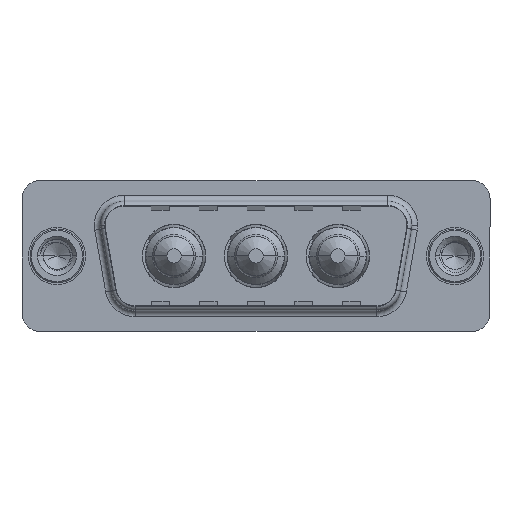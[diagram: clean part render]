
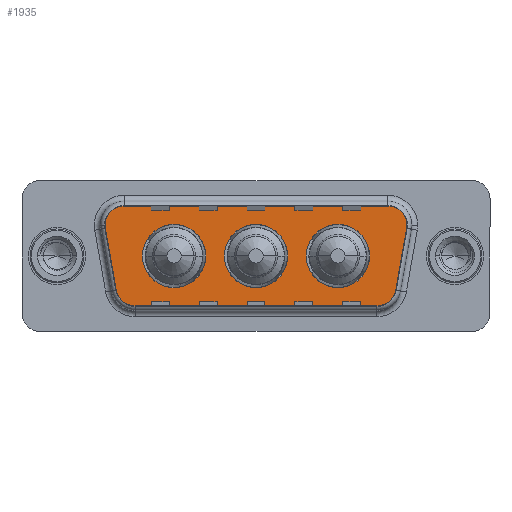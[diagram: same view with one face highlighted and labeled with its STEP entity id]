
A CAD part, top view. The second image highlights one B-rep face of the part: STEP entity #1935.
In plain terms, the highlighted planar face has unit normal (0, 0, 1).
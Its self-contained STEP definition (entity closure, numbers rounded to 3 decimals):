
#6 = VERTEX_POINT ( 'NONE', #1034 ) ;
#29 = ORIENTED_EDGE ( 'NONE', *, *, #5355, .T. ) ;
#164 = ORIENTED_EDGE ( 'NONE', *, *, #4156, .F. ) ;
#382 = EDGE_CURVE ( 'NONE', #2594, #4807, #12062, .T. ) ;
#663 = AXIS2_PLACEMENT_3D ( 'NONE', #7230, #15959, #8486 ) ;
#745 = ORIENTED_EDGE ( 'NONE', *, *, #11146, .T. ) ;
#750 = FACE_BOUND ( 'NONE', #5321, .T. ) ;
#793 = CARTESIAN_POINT ( 'NONE',  ( 29.859, 2.553, 0. ) ) ;
#1022 = CIRCLE ( 'NONE', #11190, 2.65 ) ;
#1034 = CARTESIAN_POINT ( 'NONE',  ( 19.3, 0., 0. ) ) ;
#1224 = EDGE_CURVE ( 'NONE', #3193, #6191, #15080, .T. ) ;
#1246 = DIRECTION ( 'NONE',  ( 0., 0., 1. ) ) ;
#1613 = CARTESIAN_POINT ( 'NONE',  ( 9.8, 0., 0. ) ) ;
#1647 = DIRECTION ( 'NONE',  ( -1., 0., 0. ) ) ;
#1658 = CARTESIAN_POINT ( 'NONE',  ( 16.65, 0., 0. ) ) ;
#1691 = VECTOR ( 'NONE', #12616, 1000. ) ;
#1693 = DIRECTION ( 'NONE',  ( 1., 0., 0. ) ) ;
#1715 = CARTESIAN_POINT ( 'NONE',  ( 6.434, -2.9, 0. ) ) ;
#1935 = ADVANCED_FACE ( 'NONE', ( #750, #4996, #11005, #13918 ), #15653, .T. ) ;
#2195 = CARTESIAN_POINT ( 'NONE',  ( 5.411, 2.9, 0. ) ) ;
#2594 = VERTEX_POINT ( 'NONE', #4792 ) ;
#2639 = VERTEX_POINT ( 'NONE', #12435 ) ;
#2667 = ORIENTED_EDGE ( 'NONE', *, *, #382, .T. ) ;
#2906 = DIRECTION ( 'NONE',  ( 1., 0., 0. ) ) ;
#2926 = CIRCLE ( 'NONE', #663, 2.65 ) ;
#2974 = ORIENTED_EDGE ( 'NONE', *, *, #1224, .T. ) ;
#3021 = EDGE_CURVE ( 'NONE', #6468, #2594, #11612, .T. ) ;
#3032 = DIRECTION ( 'NONE',  ( -1., 0., 0. ) ) ;
#3085 = CARTESIAN_POINT ( 'NONE',  ( 23.5, 0., 0. ) ) ;
#3167 = VERTEX_POINT ( 'NONE', #7704 ) ;
#3189 = CARTESIAN_POINT ( 'NONE',  ( 23.5, 0., 0. ) ) ;
#3193 = VERTEX_POINT ( 'NONE', #12414 ) ;
#3243 = EDGE_LOOP ( 'NONE', ( #8648, #11175 ) ) ;
#3401 = CARTESIAN_POINT ( 'NONE',  ( 6.434, -4.9, 0. ) ) ;
#3408 = CARTESIAN_POINT ( 'NONE',  ( 20.85, 0., 0. ) ) ;
#3487 = DIRECTION ( 'NONE',  ( 1., 0., 0. ) ) ;
#3648 = CARTESIAN_POINT ( 'NONE',  ( 26.866, -2.9, 0. ) ) ;
#3726 = ORIENTED_EDGE ( 'NONE', *, *, #3021, .T. ) ;
#3740 = DIRECTION ( 'NONE',  ( 1., 0., 0. ) ) ;
#3808 = AXIS2_PLACEMENT_3D ( 'NONE', #2195, #11163, #3487 ) ;
#3938 = EDGE_LOOP ( 'NONE', ( #3726, #2667, #745, #2974, #15783, #15108, #29, #9210, #5083 ) ) ;
#4156 = EDGE_CURVE ( 'NONE', #6, #4825, #15232, .T. ) ;
#4379 = DIRECTION ( 'NONE',  ( 1., 0., 0. ) ) ;
#4480 = DIRECTION ( 'NONE',  ( 1., 0., 0. ) ) ;
#4767 = VERTEX_POINT ( 'NONE', #15723 ) ;
#4792 = CARTESIAN_POINT ( 'NONE',  ( 28.836, -3.247, 0. ) ) ;
#4807 = VERTEX_POINT ( 'NONE', #793 ) ;
#4825 = VERTEX_POINT ( 'NONE', #14793 ) ;
#4984 = CARTESIAN_POINT ( 'NONE',  ( 6.434, -4.9, 0. ) ) ;
#4996 = FACE_BOUND ( 'NONE', #14342, .T. ) ;
#5043 = CARTESIAN_POINT ( 'NONE',  ( 27.889, 2.9, 0. ) ) ;
#5083 = ORIENTED_EDGE ( 'NONE', *, *, #11165, .T. ) ;
#5124 = LINE ( 'NONE', #11335, #1691 ) ;
#5321 = EDGE_LOOP ( 'NONE', ( #164, #16284 ) ) ;
#5355 = EDGE_CURVE ( 'NONE', #2639, #13304, #5124, .T. ) ;
#5622 = CIRCLE ( 'NONE', #8593, 2.65 ) ;
#5738 = DIRECTION ( 'NONE',  ( 0.174, 0.985, 0. ) ) ;
#5825 = CARTESIAN_POINT ( 'NONE',  ( 26.866, -4.9, 0. ) ) ;
#5869 = AXIS2_PLACEMENT_3D ( 'NONE', #1658, #13977, #13877 ) ;
#6157 = CARTESIAN_POINT ( 'NONE',  ( 16.65, 0., 0. ) ) ;
#6191 = VERTEX_POINT ( 'NONE', #12926 ) ;
#6260 = ORIENTED_EDGE ( 'NONE', *, *, #7836, .F. ) ;
#6334 = DIRECTION ( 'NONE',  ( -1., 0., 0. ) ) ;
#6335 = VERTEX_POINT ( 'NONE', #12010 ) ;
#6468 = VERTEX_POINT ( 'NONE', #5825 ) ;
#6509 = VERTEX_POINT ( 'NONE', #3408 ) ;
#6524 = CARTESIAN_POINT ( 'NONE',  ( 26.866, -2.9, 0. ) ) ;
#6906 = CIRCLE ( 'NONE', #15013, 2.65 ) ;
#6947 = DIRECTION ( 'NONE',  ( 0., 0., 1. ) ) ;
#7230 = CARTESIAN_POINT ( 'NONE',  ( 9.8, 0., 0. ) ) ;
#7366 = LINE ( 'NONE', #4984, #13691 ) ;
#7403 = EDGE_CURVE ( 'NONE', #6191, #4767, #14151, .T. ) ;
#7454 = DIRECTION ( 'NONE',  ( 1., 0., 0. ) ) ;
#7704 = CARTESIAN_POINT ( 'NONE',  ( 12.45, 0., 0. ) ) ;
#7747 = CARTESIAN_POINT ( 'NONE',  ( 4.464, -3.247, 0. ) ) ;
#7836 = EDGE_CURVE ( 'NONE', #6509, #12329, #5622, .T. ) ;
#7863 = AXIS2_PLACEMENT_3D ( 'NONE', #3648, #1246, #1693 ) ;
#8486 = DIRECTION ( 'NONE',  ( 1., 0., 0. ) ) ;
#8502 = CARTESIAN_POINT ( 'NONE',  ( 29.859, 2.553, 0. ) ) ;
#8593 = AXIS2_PLACEMENT_3D ( 'NONE', #3189, #12156, #4480 ) ;
#8648 = ORIENTED_EDGE ( 'NONE', *, *, #11596, .F. ) ;
#9058 = VECTOR ( 'NONE', #5738, 1000. ) ;
#9206 = AXIS2_PLACEMENT_3D ( 'NONE', #6524, #11009, #16078 ) ;
#9210 = ORIENTED_EDGE ( 'NONE', *, *, #15912, .T. ) ;
#9809 = VERTEX_POINT ( 'NONE', #3401 ) ;
#10577 = DIRECTION ( 'NONE',  ( 0., 0., 1. ) ) ;
#10643 = CARTESIAN_POINT ( 'NONE',  ( 26.15, 0., 0. ) ) ;
#10671 = AXIS2_PLACEMENT_3D ( 'NONE', #1715, #10700, #3032 ) ;
#10700 = DIRECTION ( 'NONE',  ( 0., 0., 1. ) ) ;
#10840 = VECTOR ( 'NONE', #12672, 1000. ) ;
#11005 = FACE_BOUND ( 'NONE', #3243, .T. ) ;
#11009 = DIRECTION ( 'NONE',  ( 0., 0., 1. ) ) ;
#11146 = EDGE_CURVE ( 'NONE', #4807, #3193, #11159, .T. ) ;
#11159 = CIRCLE ( 'NONE', #12802, 2. ) ;
#11163 = DIRECTION ( 'NONE',  ( 0., 0., 1. ) ) ;
#11165 = EDGE_CURVE ( 'NONE', #9809, #6468, #7366, .T. ) ;
#11175 = ORIENTED_EDGE ( 'NONE', *, *, #14110, .F. ) ;
#11190 = AXIS2_PLACEMENT_3D ( 'NONE', #1613, #10577, #2906 ) ;
#11335 = CARTESIAN_POINT ( 'NONE',  ( 3.441, 2.553, 0. ) ) ;
#11402 = CARTESIAN_POINT ( 'NONE',  ( 5.411, 4.9, 0. ) ) ;
#11596 = EDGE_CURVE ( 'NONE', #3167, #6335, #2926, .T. ) ;
#11612 = CIRCLE ( 'NONE', #9206, 2. ) ;
#11948 = EDGE_CURVE ( 'NONE', #4767, #2639, #14634, .T. ) ;
#12010 = CARTESIAN_POINT ( 'NONE',  ( 7.15, 0., 0. ) ) ;
#12062 = LINE ( 'NONE', #8502, #9058 ) ;
#12064 = DIRECTION ( 'NONE',  ( 0., 0., 1. ) ) ;
#12156 = DIRECTION ( 'NONE',  ( 0., 0., 1. ) ) ;
#12329 = VERTEX_POINT ( 'NONE', #10643 ) ;
#12378 = AXIS2_PLACEMENT_3D ( 'NONE', #3085, #12064, #4379 ) ;
#12414 = CARTESIAN_POINT ( 'NONE',  ( 29.889, 2.9, 0. ) ) ;
#12435 = CARTESIAN_POINT ( 'NONE',  ( 3.441, 2.553, 0. ) ) ;
#12616 = DIRECTION ( 'NONE',  ( 0.174, -0.985, 0. ) ) ;
#12672 = DIRECTION ( 'NONE',  ( -1., 0., 0. ) ) ;
#12802 = AXIS2_PLACEMENT_3D ( 'NONE', #5043, #13910, #6334 ) ;
#12926 = CARTESIAN_POINT ( 'NONE',  ( 27.889, 4.9, 0. ) ) ;
#13304 = VERTEX_POINT ( 'NONE', #7747 ) ;
#13425 = CARTESIAN_POINT ( 'NONE',  ( 27.889, 2.9, 0. ) ) ;
#13691 = VECTOR ( 'NONE', #3740, 1000. ) ;
#13877 = DIRECTION ( 'NONE',  ( 1., 0., 0. ) ) ;
#13910 = DIRECTION ( 'NONE',  ( 0., 0., 1. ) ) ;
#13918 = FACE_OUTER_BOUND ( 'NONE', #3938, .T. ) ;
#13960 = CIRCLE ( 'NONE', #12378, 2.65 ) ;
#13977 = DIRECTION ( 'NONE',  ( 0., 0., 1. ) ) ;
#14110 = EDGE_CURVE ( 'NONE', #6335, #3167, #1022, .T. ) ;
#14151 = LINE ( 'NONE', #11402, #10840 ) ;
#14342 = EDGE_LOOP ( 'NONE', ( #15192, #6260 ) ) ;
#14523 = EDGE_CURVE ( 'NONE', #4825, #6, #6906, .T. ) ;
#14634 = CIRCLE ( 'NONE', #3808, 2. ) ;
#14793 = CARTESIAN_POINT ( 'NONE',  ( 14., 0., 0. ) ) ;
#14972 = DIRECTION ( 'NONE',  ( 0., 0., 1. ) ) ;
#15013 = AXIS2_PLACEMENT_3D ( 'NONE', #6157, #14972, #7454 ) ;
#15080 = CIRCLE ( 'NONE', #15560, 2. ) ;
#15104 = CIRCLE ( 'NONE', #10671, 2. ) ;
#15108 = ORIENTED_EDGE ( 'NONE', *, *, #11948, .T. ) ;
#15192 = ORIENTED_EDGE ( 'NONE', *, *, #15967, .F. ) ;
#15232 = CIRCLE ( 'NONE', #5869, 2.65 ) ;
#15560 = AXIS2_PLACEMENT_3D ( 'NONE', #13425, #6947, #1647 ) ;
#15653 = PLANE ( 'NONE',  #7863 ) ;
#15723 = CARTESIAN_POINT ( 'NONE',  ( 5.411, 4.9, 0. ) ) ;
#15783 = ORIENTED_EDGE ( 'NONE', *, *, #7403, .T. ) ;
#15912 = EDGE_CURVE ( 'NONE', #13304, #9809, #15104, .T. ) ;
#15959 = DIRECTION ( 'NONE',  ( 0., 0., 1. ) ) ;
#15967 = EDGE_CURVE ( 'NONE', #12329, #6509, #13960, .T. ) ;
#16078 = DIRECTION ( 'NONE',  ( 1., 0., 0. ) ) ;
#16284 = ORIENTED_EDGE ( 'NONE', *, *, #14523, .F. ) ;
